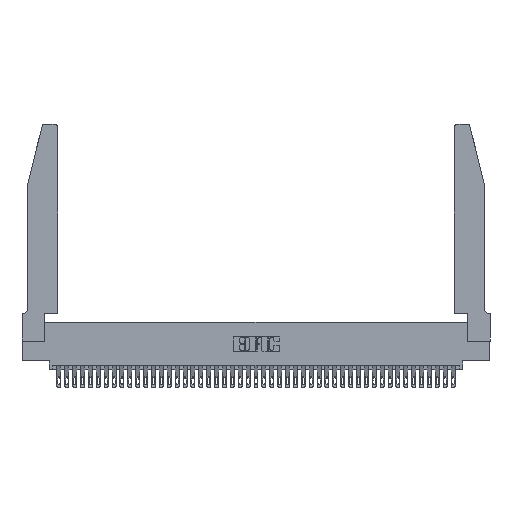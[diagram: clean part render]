
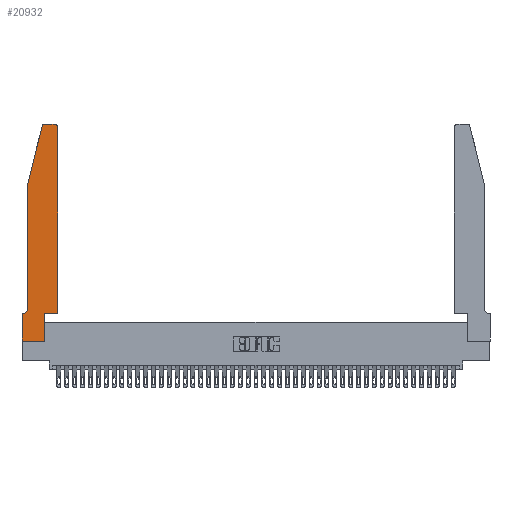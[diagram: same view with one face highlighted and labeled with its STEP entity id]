
A CAD part, top view. The second image highlights one B-rep face of the part: STEP entity #20932.
In plain terms, the highlighted planar face has unit normal (0, 0, 1).
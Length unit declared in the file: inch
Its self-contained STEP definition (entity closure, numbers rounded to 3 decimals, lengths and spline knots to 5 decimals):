
#367 = FACE_OUTER_BOUND ( 'NONE', #3600, .T. ) ;
#1181 = CARTESIAN_POINT ( 'NONE',  ( 0.4205, 2.72, 0.37 ) ) ;
#1836 = AXIS2_PLACEMENT_3D ( 'NONE', #1181, #28011, #42940 ) ;
#2093 = ORIENTED_EDGE ( 'NONE', *, *, #10731, .T. ) ;
#2194 = DIRECTION ( 'NONE',  ( 0., 0., -1. ) ) ;
#3577 = VECTOR ( 'NONE', #7514, 39.37008 ) ;
#3600 = EDGE_LOOP ( 'NONE', ( #32969, #12127, #19969, #38286, #2093, #11895, #9318, #30117, #27107, #20345, #33191, #28745 ) ) ;
#3634 = LINE ( 'NONE', #34332, #32894 ) ;
#3688 = DIRECTION ( 'NONE',  ( -0.239, -0.971, 0. ) ) ;
#4856 = CARTESIAN_POINT ( 'NONE',  ( 0., 0., 0.37 ) ) ;
#5091 = LINE ( 'NONE', #22722, #25243 ) ;
#5189 = CARTESIAN_POINT ( 'NONE',  ( 0.4505, 0.35, 0.37 ) ) ;
#5273 = VECTOR ( 'NONE', #40999, 39.37008 ) ;
#5666 = EDGE_CURVE ( 'NONE', #32450, #19093, #43555, .T. ) ;
#6644 = AXIS2_PLACEMENT_3D ( 'NONE', #32467, #2194, #25891 ) ;
#7004 = EDGE_CURVE ( 'NONE', #7277, #27205, #5091, .T. ) ;
#7199 = DIRECTION ( 'NONE',  ( 1., 0., 0. ) ) ;
#7277 = VERTEX_POINT ( 'NONE', #42261 ) ;
#7369 = LINE ( 'NONE', #27154, #5273 ) ;
#7514 = DIRECTION ( 'NONE',  ( 0., -1., 0. ) ) ;
#7612 = CARTESIAN_POINT ( 'NONE',  ( 0.2865, 0., 0.37 ) ) ;
#8395 = EDGE_CURVE ( 'NONE', #33000, #8654, #23100, .T. ) ;
#8654 = VERTEX_POINT ( 'NONE', #19496 ) ;
#9318 = ORIENTED_EDGE ( 'NONE', *, *, #38295, .T. ) ;
#9996 = DIRECTION ( 'NONE',  ( 1., 0., 0. ) ) ;
#10731 = EDGE_CURVE ( 'NONE', #24073, #12763, #36451, .T. ) ;
#11895 = ORIENTED_EDGE ( 'NONE', *, *, #25307, .T. ) ;
#12127 = ORIENTED_EDGE ( 'NONE', *, *, #14875, .T. ) ;
#12763 = VERTEX_POINT ( 'NONE', #14759 ) ;
#13080 = VERTEX_POINT ( 'NONE', #4856 ) ;
#13884 = CARTESIAN_POINT ( 'NONE',  ( 0.2605, 2.75, 0.37 ) ) ;
#14034 = VECTOR ( 'NONE', #30689, 39.37008 ) ;
#14759 = CARTESIAN_POINT ( 'NONE',  ( 0.0055, 0.35, 0.37 ) ) ;
#14875 = EDGE_CURVE ( 'NONE', #8654, #7277, #31307, .T. ) ;
#15285 = LINE ( 'NONE', #16411, #20546 ) ;
#15333 = EDGE_CURVE ( 'NONE', #27822, #32450, #16368, .T. ) ;
#15633 = DIRECTION ( 'NONE',  ( 1., 0., 0. ) ) ;
#15778 = PLANE ( 'NONE',  #40877 ) ;
#16368 = LINE ( 'NONE', #38771, #25924 ) ;
#16411 = CARTESIAN_POINT ( 'NONE',  ( 0., 0., 0.37 ) ) ;
#16530 = DIRECTION ( 'NONE',  ( 1., 0., 0. ) ) ;
#16735 = CARTESIAN_POINT ( 'NONE',  ( 0.4505, 2.72, 0.37 ) ) ;
#17443 = DIRECTION ( 'NONE',  ( 0., 0., 1. ) ) ;
#17591 = CARTESIAN_POINT ( 'NONE',  ( 0.284, 2.72, 0.37 ) ) ;
#18159 = LINE ( 'NONE', #5189, #33035 ) ;
#19093 = VERTEX_POINT ( 'NONE', #35264 ) ;
#19318 = DIRECTION ( 'NONE',  ( 0., 0., 1. ) ) ;
#19496 = CARTESIAN_POINT ( 'NONE',  ( 0.284, 2.75, 0.37 ) ) ;
#19969 = ORIENTED_EDGE ( 'NONE', *, *, #7004, .T. ) ;
#20345 = ORIENTED_EDGE ( 'NONE', *, *, #5666, .T. ) ;
#20546 = VECTOR ( 'NONE', #9996, 39.37008 ) ;
#20717 = CARTESIAN_POINT ( 'NONE',  ( 0., 0.35, 0.37 ) ) ;
#20932 = ADVANCED_FACE ( 'NONE', ( #367 ), #15778, .T. ) ;
#22722 = CARTESIAN_POINT ( 'NONE',  ( 0.0755, 2., 0.37 ) ) ;
#22889 = CARTESIAN_POINT ( 'NONE',  ( 0.0755, 2., 0.37 ) ) ;
#23100 = LINE ( 'NONE', #13884, #14034 ) ;
#24073 = VERTEX_POINT ( 'NONE', #29024 ) ;
#24237 = LINE ( 'NONE', #34699, #3577 ) ;
#24492 = DIRECTION ( 'NONE',  ( -1., 0., 0. ) ) ;
#24712 = VERTEX_POINT ( 'NONE', #16735 ) ;
#25243 = VECTOR ( 'NONE', #3688, 39.37008 ) ;
#25307 = EDGE_CURVE ( 'NONE', #12763, #42966, #3634, .T. ) ;
#25891 = DIRECTION ( 'NONE',  ( -1., 0., 0. ) ) ;
#25924 = VECTOR ( 'NONE', #28446, 39.37008 ) ;
#26897 = AXIS2_PLACEMENT_3D ( 'NONE', #17591, #17443, #7199 ) ;
#27107 = ORIENTED_EDGE ( 'NONE', *, *, #15333, .T. ) ;
#27154 = CARTESIAN_POINT ( 'NONE',  ( 0.0755, 2., 0.37 ) ) ;
#27205 = VERTEX_POINT ( 'NONE', #22889 ) ;
#27822 = VERTEX_POINT ( 'NONE', #7612 ) ;
#28011 = DIRECTION ( 'NONE',  ( 0., 0., 1. ) ) ;
#28064 = VECTOR ( 'NONE', #16530, 39.37008 ) ;
#28446 = DIRECTION ( 'NONE',  ( 0., 1., 0. ) ) ;
#28745 = ORIENTED_EDGE ( 'NONE', *, *, #41837, .T. ) ;
#29024 = CARTESIAN_POINT ( 'NONE',  ( 0.0755, 0.42, 0.37 ) ) ;
#29447 = CARTESIAN_POINT ( 'NONE',  ( 0., 0.35, 0.37 ) ) ;
#30037 = CARTESIAN_POINT ( 'NONE',  ( 0.4505, 0.35, 0.37 ) ) ;
#30117 = ORIENTED_EDGE ( 'NONE', *, *, #38730, .T. ) ;
#30689 = DIRECTION ( 'NONE',  ( -1., 0., 0. ) ) ;
#31307 = CIRCLE ( 'NONE', #26897, 0.03 ) ;
#32212 = DIRECTION ( 'NONE',  ( 0., 1., 0. ) ) ;
#32450 = VERTEX_POINT ( 'NONE', #42195 ) ;
#32467 = CARTESIAN_POINT ( 'NONE',  ( 0.0055, 0.42, 0.37 ) ) ;
#32894 = VECTOR ( 'NONE', #24492, 39.37008 ) ;
#32969 = ORIENTED_EDGE ( 'NONE', *, *, #8395, .T. ) ;
#33000 = VERTEX_POINT ( 'NONE', #39724 ) ;
#33035 = VECTOR ( 'NONE', #32212, 39.37008 ) ;
#33191 = ORIENTED_EDGE ( 'NONE', *, *, #35875, .T. ) ;
#34332 = CARTESIAN_POINT ( 'NONE',  ( 0.0755, 0.35, 0.37 ) ) ;
#34699 = CARTESIAN_POINT ( 'NONE',  ( 0., 0., 0.37 ) ) ;
#35264 = CARTESIAN_POINT ( 'NONE',  ( 0.4505, 0.35, 0.37 ) ) ;
#35875 = EDGE_CURVE ( 'NONE', #19093, #24712, #18159, .T. ) ;
#36451 = CIRCLE ( 'NONE', #6644, 0.07 ) ;
#38286 = ORIENTED_EDGE ( 'NONE', *, *, #40381, .T. ) ;
#38295 = EDGE_CURVE ( 'NONE', #42966, #13080, #24237, .T. ) ;
#38730 = EDGE_CURVE ( 'NONE', #13080, #27822, #15285, .T. ) ;
#38771 = CARTESIAN_POINT ( 'NONE',  ( 0.2865, 0.35, 0.37 ) ) ;
#39724 = CARTESIAN_POINT ( 'NONE',  ( 0.4205, 2.75, 0.37 ) ) ;
#39757 = CIRCLE ( 'NONE', #1836, 0.03 ) ;
#40381 = EDGE_CURVE ( 'NONE', #27205, #24073, #7369, .T. ) ;
#40877 = AXIS2_PLACEMENT_3D ( 'NONE', #29447, #19318, #15633 ) ;
#40999 = DIRECTION ( 'NONE',  ( 0., -1., 0. ) ) ;
#41837 = EDGE_CURVE ( 'NONE', #24712, #33000, #39757, .T. ) ;
#42195 = CARTESIAN_POINT ( 'NONE',  ( 0.2865, 0.35, 0.37 ) ) ;
#42261 = CARTESIAN_POINT ( 'NONE',  ( 0.25487, 2.72718, 0.37 ) ) ;
#42940 = DIRECTION ( 'NONE',  ( 1., 0., 0. ) ) ;
#42966 = VERTEX_POINT ( 'NONE', #20717 ) ;
#43555 = LINE ( 'NONE', #30037, #28064 ) ;
